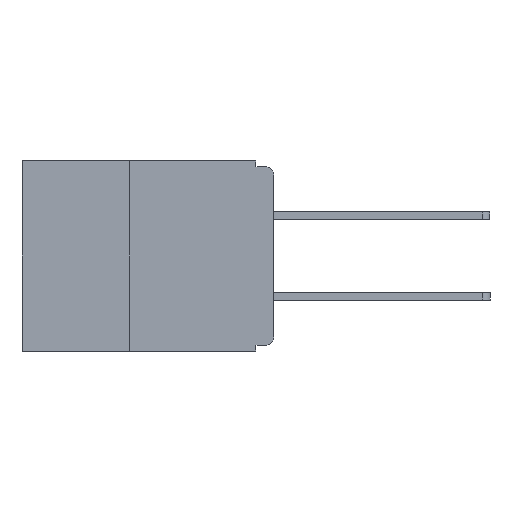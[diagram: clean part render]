
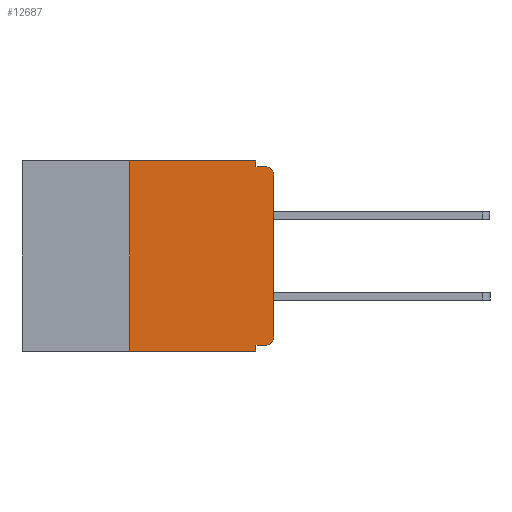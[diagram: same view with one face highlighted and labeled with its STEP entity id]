
A CAD part, left-side view. The second image highlights one B-rep face of the part: STEP entity #12687.
In plain terms, the highlighted planar face has unit normal (-1, 0, 0).
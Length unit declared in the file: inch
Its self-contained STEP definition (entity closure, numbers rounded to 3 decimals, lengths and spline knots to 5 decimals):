
#297 = VECTOR ( 'NONE', #10652, 39.37008 ) ;
#943 = EDGE_CURVE ( 'NONE', #23058, #28519, #4284, .T. ) ;
#985 = AXIS2_PLACEMENT_3D ( 'NONE', #19432, #19407, #19401 ) ;
#1267 = VERTEX_POINT ( 'NONE', #25022 ) ;
#1444 = EDGE_CURVE ( 'NONE', #17147, #14394, #8980, .T. ) ;
#1841 = AXIS2_PLACEMENT_3D ( 'NONE', #6767, #23784, #9274 ) ;
#1979 = PLANE ( 'NONE',  #25577 ) ;
#2562 = ORIENTED_EDGE ( 'NONE', *, *, #23376, .T. ) ;
#3032 = CARTESIAN_POINT ( 'NONE',  ( 0., 0., -0.01 ) ) ;
#3120 = ORIENTED_EDGE ( 'NONE', *, *, #9190, .F. ) ;
#4284 = LINE ( 'NONE', #6614, #22989 ) ;
#4317 = EDGE_CURVE ( 'NONE', #1267, #28519, #12905, .T. ) ;
#4521 = DIRECTION ( 'NONE',  ( 1., 0., 0. ) ) ;
#4923 = CARTESIAN_POINT ( 'NONE',  ( 0., 0.031, 0. ) ) ;
#4925 = ORIENTED_EDGE ( 'NONE', *, *, #29306, .F. ) ;
#4978 = LINE ( 'NONE', #4923, #23633 ) ;
#6138 = LINE ( 'NONE', #9499, #18393 ) ;
#6569 = CARTESIAN_POINT ( 'NONE',  ( 0., 0., -0.305 ) ) ;
#6614 = CARTESIAN_POINT ( 'NONE',  ( 0., 0.031, -0.33 ) ) ;
#6767 = CARTESIAN_POINT ( 'NONE',  ( 0., 0.015, -0.305 ) ) ;
#7607 = CARTESIAN_POINT ( 'NONE',  ( 0., 0.031, -0.01 ) ) ;
#7674 = CARTESIAN_POINT ( 'NONE',  ( 0., 0.031, -0.33 ) ) ;
#7917 = VERTEX_POINT ( 'NONE', #7607 ) ;
#8668 = DIRECTION ( 'NONE',  ( 0., 0., -1. ) ) ;
#8867 = VECTOR ( 'NONE', #23333, 39.37008 ) ;
#8932 = CARTESIAN_POINT ( 'NONE',  ( 0., 0.437, 0. ) ) ;
#8980 = CIRCLE ( 'NONE', #985, 0.015 ) ;
#9190 = EDGE_CURVE ( 'NONE', #7917, #14394, #9844, .T. ) ;
#9274 = DIRECTION ( 'NONE',  ( 0., 0., -1. ) ) ;
#9499 = CARTESIAN_POINT ( 'NONE',  ( 0., 0., -0.32 ) ) ;
#9844 = LINE ( 'NONE', #3032, #27626 ) ;
#10203 = LINE ( 'NONE', #8932, #15950 ) ;
#10652 = DIRECTION ( 'NONE',  ( 0., 0., 1. ) ) ;
#11199 = CARTESIAN_POINT ( 'NONE',  ( 0., 0.437, -0.33 ) ) ;
#11441 = EDGE_CURVE ( 'NONE', #12606, #23058, #6138, .T. ) ;
#11497 = DIRECTION ( 'NONE',  ( 0., -1., 0. ) ) ;
#11681 = EDGE_LOOP ( 'NONE', ( #26048, #21160, #3120, #14400, #4925, #28896, #16832, #19103, #14207, #2562 ) ) ;
#12283 = CARTESIAN_POINT ( 'NONE',  ( 0., 0., -0.025 ) ) ;
#12606 = VERTEX_POINT ( 'NONE', #13928 ) ;
#12687 = ADVANCED_FACE ( 'NONE', ( #14973 ), #1979, .F. ) ;
#12731 = CARTESIAN_POINT ( 'NONE',  ( 0., 0.031, -0.32 ) ) ;
#12905 = LINE ( 'NONE', #11199, #18581 ) ;
#13928 = CARTESIAN_POINT ( 'NONE',  ( 0., 0.015, -0.32 ) ) ;
#14207 = ORIENTED_EDGE ( 'NONE', *, *, #11441, .F. ) ;
#14394 = VERTEX_POINT ( 'NONE', #30770 ) ;
#14400 = ORIENTED_EDGE ( 'NONE', *, *, #20719, .F. ) ;
#14973 = FACE_OUTER_BOUND ( 'NONE', #11681, .T. ) ;
#15950 = VECTOR ( 'NONE', #21049, 39.37008 ) ;
#16120 = CARTESIAN_POINT ( 'NONE',  ( 0., 0.25, -0.33 ) ) ;
#16150 = LINE ( 'NONE', #16120, #8867 ) ;
#16658 = CARTESIAN_POINT ( 'NONE',  ( 0., 0.437, 0. ) ) ;
#16832 = ORIENTED_EDGE ( 'NONE', *, *, #4317, .T. ) ;
#16926 = VERTEX_POINT ( 'NONE', #6569 ) ;
#17147 = VERTEX_POINT ( 'NONE', #12283 ) ;
#17484 = EDGE_CURVE ( 'NONE', #1267, #21942, #16150, .T. ) ;
#17786 = DIRECTION ( 'NONE',  ( 0., -1., 0. ) ) ;
#18393 = VECTOR ( 'NONE', #26417, 39.37008 ) ;
#18581 = VECTOR ( 'NONE', #11497, 39.37008 ) ;
#19103 = ORIENTED_EDGE ( 'NONE', *, *, #943, .F. ) ;
#19319 = VERTEX_POINT ( 'NONE', #30631 ) ;
#19401 = DIRECTION ( 'NONE',  ( 0., 0., -1. ) ) ;
#19407 = DIRECTION ( 'NONE',  ( -1., 0., 0. ) ) ;
#19432 = CARTESIAN_POINT ( 'NONE',  ( 0., 0.015, -0.025 ) ) ;
#19577 = DIRECTION ( 'NONE',  ( 0., 0., -1. ) ) ;
#20719 = EDGE_CURVE ( 'NONE', #19319, #7917, #4978, .T. ) ;
#20723 = CARTESIAN_POINT ( 'NONE',  ( 0., 0.25, 0. ) ) ;
#21049 = DIRECTION ( 'NONE',  ( 0., -1., 0. ) ) ;
#21160 = ORIENTED_EDGE ( 'NONE', *, *, #1444, .T. ) ;
#21615 = DIRECTION ( 'NONE',  ( 0., 0., -1. ) ) ;
#21942 = VERTEX_POINT ( 'NONE', #20723 ) ;
#21982 = CIRCLE ( 'NONE', #1841, 0.015 ) ;
#22232 = LINE ( 'NONE', #22710, #297 ) ;
#22710 = CARTESIAN_POINT ( 'NONE',  ( 0., 0., 0. ) ) ;
#22989 = VECTOR ( 'NONE', #8668, 39.37008 ) ;
#23058 = VERTEX_POINT ( 'NONE', #12731 ) ;
#23333 = DIRECTION ( 'NONE',  ( 0., 0., 1. ) ) ;
#23376 = EDGE_CURVE ( 'NONE', #12606, #16926, #21982, .T. ) ;
#23633 = VECTOR ( 'NONE', #19577, 39.37008 ) ;
#23784 = DIRECTION ( 'NONE',  ( -1., 0., 0. ) ) ;
#25022 = CARTESIAN_POINT ( 'NONE',  ( 0., 0.25, -0.33 ) ) ;
#25423 = EDGE_CURVE ( 'NONE', #16926, #17147, #22232, .T. ) ;
#25577 = AXIS2_PLACEMENT_3D ( 'NONE', #16658, #4521, #21615 ) ;
#26048 = ORIENTED_EDGE ( 'NONE', *, *, #25423, .T. ) ;
#26417 = DIRECTION ( 'NONE',  ( 0., 1., 0. ) ) ;
#27626 = VECTOR ( 'NONE', #17786, 39.37008 ) ;
#28519 = VERTEX_POINT ( 'NONE', #7674 ) ;
#28896 = ORIENTED_EDGE ( 'NONE', *, *, #17484, .F. ) ;
#29306 = EDGE_CURVE ( 'NONE', #21942, #19319, #10203, .T. ) ;
#30631 = CARTESIAN_POINT ( 'NONE',  ( 0., 0.031, 0. ) ) ;
#30770 = CARTESIAN_POINT ( 'NONE',  ( 0., 0.015, -0.01 ) ) ;
